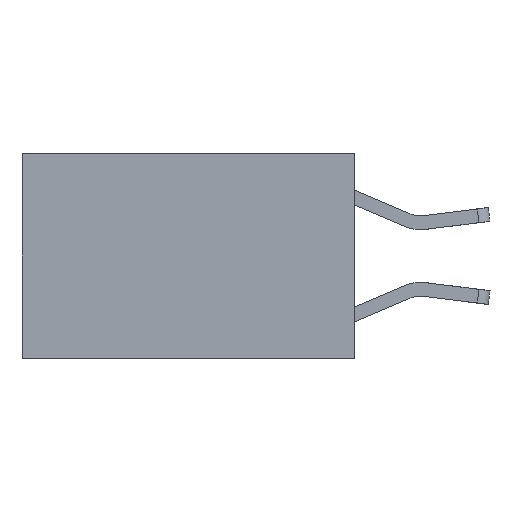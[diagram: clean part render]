
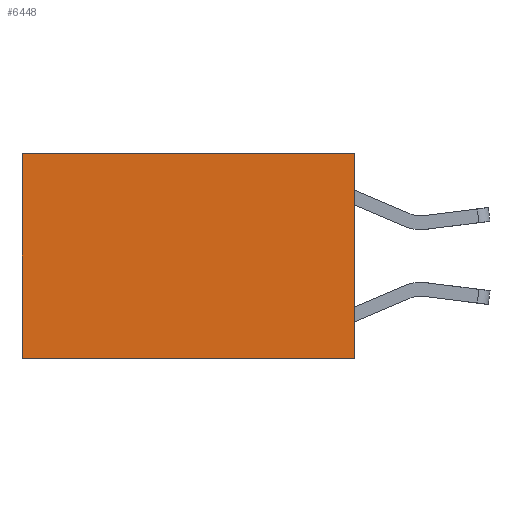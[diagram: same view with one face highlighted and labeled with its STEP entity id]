
A CAD part, left-side view. The second image highlights one B-rep face of the part: STEP entity #6448.
In plain terms, the highlighted planar face has unit normal (-1, 0, 0).
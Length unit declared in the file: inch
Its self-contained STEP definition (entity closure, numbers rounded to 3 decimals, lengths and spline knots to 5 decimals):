
#209 = EDGE_CURVE ( 'NONE', #507, #4716, #7902, .T. ) ;
#507 = VERTEX_POINT ( 'NONE', #3202 ) ;
#641 = CARTESIAN_POINT ( 'NONE',  ( 0.2625, 0.6, 0. ) ) ;
#833 = ORIENTED_EDGE ( 'NONE', *, *, #2377, .T. ) ;
#1554 = VERTEX_POINT ( 'NONE', #6864 ) ;
#2295 = EDGE_CURVE ( 'NONE', #5199, #1554, #5332, .T. ) ;
#2310 = DIRECTION ( 'NONE',  ( 0., 0., -1. ) ) ;
#2319 = DIRECTION ( 'NONE',  ( 1., 0., 0. ) ) ;
#2330 = CARTESIAN_POINT ( 'NONE',  ( 0.2625, 0., 0. ) ) ;
#2370 = PLANE ( 'NONE',  #6076 ) ;
#2377 = EDGE_CURVE ( 'NONE', #4716, #1554, #5110, .T. ) ;
#2885 = FACE_OUTER_BOUND ( 'NONE', #5566, .T. ) ;
#2906 = VECTOR ( 'NONE', #3918, 39.37008 ) ;
#2914 = LINE ( 'NONE', #7427, #2906 ) ;
#3202 = CARTESIAN_POINT ( 'NONE',  ( 0.2625, 0., 0. ) ) ;
#3636 = CARTESIAN_POINT ( 'NONE',  ( 0.2625, 0., 0. ) ) ;
#3893 = EDGE_CURVE ( 'NONE', #507, #5199, #2914, .T. ) ;
#3918 = DIRECTION ( 'NONE',  ( 0., 0., -1. ) ) ;
#4561 = CARTESIAN_POINT ( 'NONE',  ( 0.2625, 0.6, 0. ) ) ;
#4716 = VERTEX_POINT ( 'NONE', #641 ) ;
#4784 = DIRECTION ( 'NONE',  ( 0., 0., -1. ) ) ;
#5008 = ORIENTED_EDGE ( 'NONE', *, *, #2295, .F. ) ;
#5016 = ORIENTED_EDGE ( 'NONE', *, *, #3893, .F. ) ;
#5092 = VECTOR ( 'NONE', #4784, 39.37008 ) ;
#5110 = LINE ( 'NONE', #4561, #5092 ) ;
#5199 = VERTEX_POINT ( 'NONE', #8047 ) ;
#5233 = ORIENTED_EDGE ( 'NONE', *, *, #209, .T. ) ;
#5304 = VECTOR ( 'NONE', #6069, 39.37008 ) ;
#5332 = LINE ( 'NONE', #5994, #5304 ) ;
#5566 = EDGE_LOOP ( 'NONE', ( #833, #5008, #5016, #5233 ) ) ;
#5994 = CARTESIAN_POINT ( 'NONE',  ( 0.2625, 0., -0.37 ) ) ;
#6069 = DIRECTION ( 'NONE',  ( 0., 1., 0. ) ) ;
#6076 = AXIS2_PLACEMENT_3D ( 'NONE', #2330, #2319, #2310 ) ;
#6448 = ADVANCED_FACE ( 'NONE', ( #2885 ), #2370, .F. ) ;
#6594 = DIRECTION ( 'NONE',  ( 0., 1., 0. ) ) ;
#6864 = CARTESIAN_POINT ( 'NONE',  ( 0.2625, 0.6, -0.37 ) ) ;
#7427 = CARTESIAN_POINT ( 'NONE',  ( 0.2625, 0., 0. ) ) ;
#7902 = LINE ( 'NONE', #3636, #7935 ) ;
#7935 = VECTOR ( 'NONE', #6594, 39.37008 ) ;
#8047 = CARTESIAN_POINT ( 'NONE',  ( 0.2625, 0., -0.37 ) ) ;
